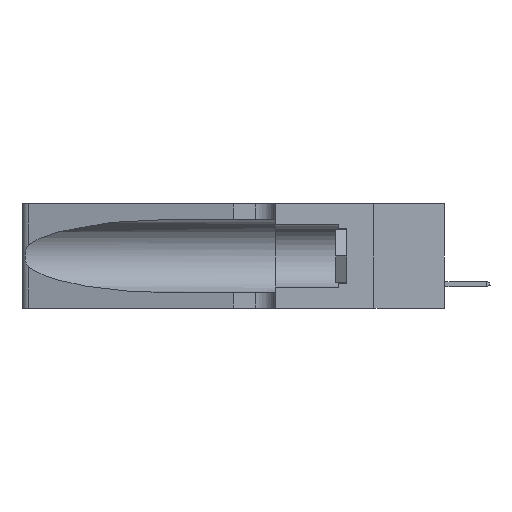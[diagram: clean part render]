
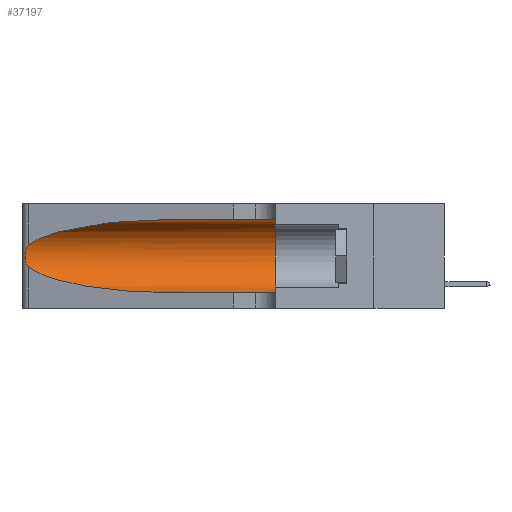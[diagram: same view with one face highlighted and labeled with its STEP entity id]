
A CAD part, left-side view. The second image highlights one B-rep face of the part: STEP entity #37197.
In plain terms, the highlighted cylindrical face has radius 3.308 mm (diameter 6.617 mm), a partial arc.
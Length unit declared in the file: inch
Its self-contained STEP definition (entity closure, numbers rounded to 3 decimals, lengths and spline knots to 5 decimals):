
#669 = CARTESIAN_POINT ( 'NONE',  ( 0.1305, 0.35, 0.05475 ) ) ;
#2205 = ORIENTED_EDGE ( 'NONE', *, *, #3492, .T. ) ;
#2335 = CARTESIAN_POINT ( 'NONE',  ( 0.26018, 1.23835, 0.19895 ) ) ;
#3492 = EDGE_CURVE ( 'NONE', #50351, #29069, #23568, .T. ) ;
#6192 = CARTESIAN_POINT ( 'NONE',  ( 0.25487, 1.22718, 0.14631 ) ) ;
#6494 = CARTESIAN_POINT ( 'NONE',  ( 0.1305, 0.35, 0.185 ) ) ;
#6602 = CARTESIAN_POINT ( 'NONE',  ( 0.25555, 1.22993, 0.14849 ) ) ;
#8412 = CARTESIAN_POINT ( 'NONE',  ( 0.25487, 1.22718, 0.22369 ) ) ;
#10470 = DIRECTION ( 'NONE',  ( 0., 0., 1. ) ) ;
#11749 = CARTESIAN_POINT ( 'NONE',  ( 0.25487, 1.22718, 0.14631 ) ) ;
#12654 = EDGE_CURVE ( 'NONE', #23341, #49177, #17189, .T. ) ;
#13072 = LINE ( 'NONE', #17980, #43797 ) ;
#14100 =( BOUNDED_CURVE ( )  B_SPLINE_CURVE ( 3, ( #24484, #24021, #48497, #24936 ),
 .UNSPECIFIED., .F., .F. ) 
 B_SPLINE_CURVE_WITH_KNOTS ( ( 4, 4 ),
 ( 1.5708, 2.84003 ),
 .UNSPECIFIED. ) 
 CURVE ( )  GEOMETRIC_REPRESENTATION_ITEM ( )  RATIONAL_B_SPLINE_CURVE ( ( 1., 0.87, 0.87, 1. ) ) 
 REPRESENTATION_ITEM ( '' )  );
#17189 = LINE ( 'NONE', #46409, #24763 ) ;
#17980 = CARTESIAN_POINT ( 'NONE',  ( 0.1305, 1.61858, 0.05475 ) ) ;
#18469 = CARTESIAN_POINT ( 'NONE',  ( 0.25555, 1.22994, 0.2215 ) ) ;
#18630 = ORIENTED_EDGE ( 'NONE', *, *, #12654, .F. ) ;
#18857 = CARTESIAN_POINT ( 'NONE',  ( 0.25856, 1.23593, 0.16098 ) ) ;
#19130 = EDGE_LOOP ( 'NONE', ( #20174, #2205, #21223, #50252, #51202, #18630 ) ) ;
#20174 = ORIENTED_EDGE ( 'NONE', *, *, #46137, .T. ) ;
#20237 = CARTESIAN_POINT ( 'NONE',  ( 0.1305, 0.35, 0.31525 ) ) ;
#21223 = ORIENTED_EDGE ( 'NONE', *, *, #45544, .T. ) ;
#22022 = DIRECTION ( 'NONE',  ( 0., -1., 0. ) ) ;
#22298 = CARTESIAN_POINT ( 'NONE',  ( 0.18966, 0.96281, 0.05475 ) ) ;
#23022 = CARTESIAN_POINT ( 'NONE',  ( 0.26075, 1.23896, 0.19203 ) ) ;
#23341 = VERTEX_POINT ( 'NONE', #44428 ) ;
#23568 = B_SPLINE_CURVE_WITH_KNOTS ( 'NONE', 3,
 ( #42920, #18469, #46908, #30155, #46162, #2335, #23022, #34356, #42743, #18857, #50414, #46547, #6602, #6192 ),
 .UNSPECIFIED., .F., .F.,
 ( 4, 2, 2, 2, 2, 2, 4 ),
 ( 0., 0.00027, 0.00053, 0.00107, 0.0016, 0.00187, 0.00214 ),
 .UNSPECIFIED. ) ;
#24021 = CARTESIAN_POINT ( 'NONE',  ( 0.18966, 0.96281, 0.31525 ) ) ;
#24484 = CARTESIAN_POINT ( 'NONE',  ( 0.1305, 0.72297, 0.31525 ) ) ;
#24763 = VECTOR ( 'NONE', #50074, 39.37008 ) ;
#24936 = CARTESIAN_POINT ( 'NONE',  ( 0.25487, 1.22718, 0.22369 ) ) ;
#25969 = DIRECTION ( 'NONE',  ( 0., -1., 0. ) ) ;
#28041 = FACE_OUTER_BOUND ( 'NONE', #19130, .T. ) ;
#28161 = EDGE_CURVE ( 'NONE', #40698, #44916, #13072, .T. ) ;
#28548 = CYLINDRICAL_SURFACE ( 'NONE', #49825, 0.13025 ) ;
#29065 = EDGE_CURVE ( 'NONE', #49177, #44916, #38692, .T. ) ;
#29069 = VERTEX_POINT ( 'NONE', #11749 ) ;
#30155 = CARTESIAN_POINT ( 'NONE',  ( 0.25787, 1.23484, 0.2124 ) ) ;
#34356 = CARTESIAN_POINT ( 'NONE',  ( 0.26075, 1.23896, 0.178 ) ) ;
#34444 = DIRECTION ( 'NONE',  ( 0., 1., 0. ) ) ;
#37197 = ADVANCED_FACE ( 'NONE', ( #28041 ), #28548, .F. ) ;
#38168 = CARTESIAN_POINT ( 'NONE',  ( 0.2373, 1.15595, 0.08982 ) ) ;
#38366 = CARTESIAN_POINT ( 'NONE',  ( 0.1305, 1.61858, 0.185 ) ) ;
#38692 = CIRCLE ( 'NONE', #47999, 0.13025 ) ;
#40698 = VERTEX_POINT ( 'NONE', #49514 ) ;
#42199 = CARTESIAN_POINT ( 'NONE',  ( 0.25487, 1.22718, 0.14631 ) ) ;
#42743 = CARTESIAN_POINT ( 'NONE',  ( 0.26017, 1.23833, 0.17102 ) ) ;
#42920 = CARTESIAN_POINT ( 'NONE',  ( 0.25487, 1.22718, 0.22369 ) ) ;
#42932 = CARTESIAN_POINT ( 'NONE',  ( 0.1305, 0.72297, 0.05475 ) ) ;
#43620 =( BOUNDED_CURVE ( )  B_SPLINE_CURVE ( 3, ( #42199, #38168, #22298, #42932 ),
 .UNSPECIFIED., .F., .T. ) 
 B_SPLINE_CURVE_WITH_KNOTS ( ( 4, 4 ),
 ( 3.44316, 4.71239 ),
 .UNSPECIFIED. ) 
 CURVE ( )  GEOMETRIC_REPRESENTATION_ITEM ( )  RATIONAL_B_SPLINE_CURVE ( ( 1., 0.87, 0.87, 1. ) ) 
 REPRESENTATION_ITEM ( '' )  );
#43797 = VECTOR ( 'NONE', #22022, 39.37008 ) ;
#44428 = CARTESIAN_POINT ( 'NONE',  ( 0.1305, 0.72297, 0.31525 ) ) ;
#44916 = VERTEX_POINT ( 'NONE', #669 ) ;
#45544 = EDGE_CURVE ( 'NONE', #29069, #40698, #43620, .T. ) ;
#46137 = EDGE_CURVE ( 'NONE', #23341, #50351, #14100, .T. ) ;
#46162 = CARTESIAN_POINT ( 'NONE',  ( 0.25854, 1.2359, 0.20912 ) ) ;
#46409 = CARTESIAN_POINT ( 'NONE',  ( 0.1305, 1.61858, 0.31525 ) ) ;
#46547 = CARTESIAN_POINT ( 'NONE',  ( 0.25639, 1.23186, 0.15144 ) ) ;
#46908 = CARTESIAN_POINT ( 'NONE',  ( 0.25639, 1.23184, 0.21858 ) ) ;
#47999 = AXIS2_PLACEMENT_3D ( 'NONE', #6494, #34444, #10470 ) ;
#48497 = CARTESIAN_POINT ( 'NONE',  ( 0.2373, 1.15595, 0.28018 ) ) ;
#49177 = VERTEX_POINT ( 'NONE', #20237 ) ;
#49514 = CARTESIAN_POINT ( 'NONE',  ( 0.1305, 0.72297, 0.05475 ) ) ;
#49642 = DIRECTION ( 'NONE',  ( 0., 0., -1. ) ) ;
#49825 = AXIS2_PLACEMENT_3D ( 'NONE', #38366, #25969, #49642 ) ;
#50074 = DIRECTION ( 'NONE',  ( 0., -1., 0. ) ) ;
#50252 = ORIENTED_EDGE ( 'NONE', *, *, #28161, .T. ) ;
#50351 = VERTEX_POINT ( 'NONE', #8412 ) ;
#50414 = CARTESIAN_POINT ( 'NONE',  ( 0.25789, 1.23486, 0.15765 ) ) ;
#51202 = ORIENTED_EDGE ( 'NONE', *, *, #29065, .F. ) ;
